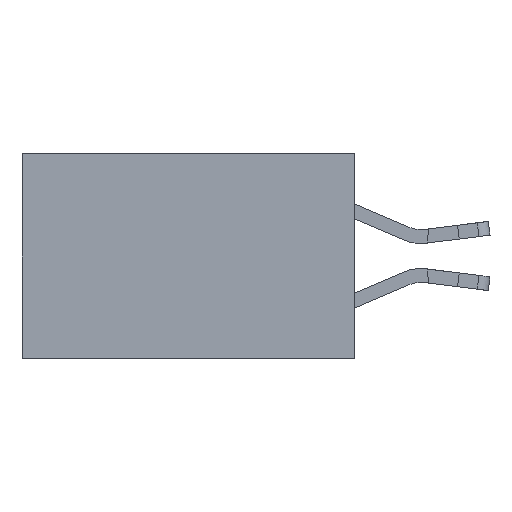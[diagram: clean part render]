
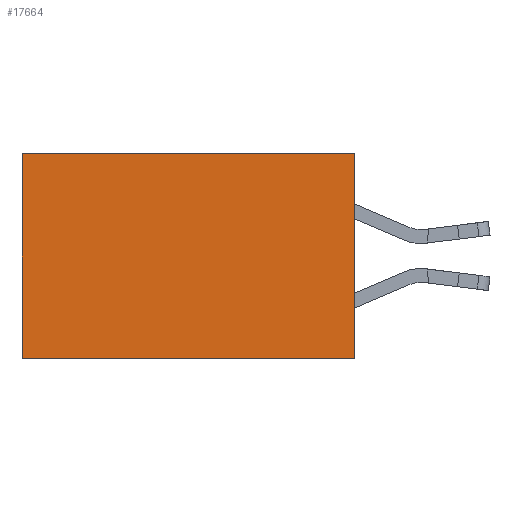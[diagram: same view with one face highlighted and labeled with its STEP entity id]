
A CAD part, left-side view. The second image highlights one B-rep face of the part: STEP entity #17664.
In plain terms, the highlighted planar face has unit normal (-1, 0, 0).
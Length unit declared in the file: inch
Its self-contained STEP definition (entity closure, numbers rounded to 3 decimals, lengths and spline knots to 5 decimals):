
#188 = VERTEX_POINT ( 'NONE', #12939 ) ;
#426 = VECTOR ( 'NONE', #7050, 39.37008 ) ;
#556 = CARTESIAN_POINT ( 'NONE',  ( 0.2615, 0., 0. ) ) ;
#1027 = EDGE_LOOP ( 'NONE', ( #6830, #12116, #4353, #14062 ) ) ;
#1072 = DIRECTION ( 'NONE',  ( 1., 0., 0. ) ) ;
#2561 = LINE ( 'NONE', #17749, #13215 ) ;
#3249 = DIRECTION ( 'NONE',  ( 0., 0., -1. ) ) ;
#3664 = EDGE_CURVE ( 'NONE', #188, #5093, #8620, .T. ) ;
#3828 = EDGE_CURVE ( 'NONE', #7345, #5093, #2561, .T. ) ;
#4353 = ORIENTED_EDGE ( 'NONE', *, *, #13419, .F. ) ;
#4537 = CARTESIAN_POINT ( 'NONE',  ( 0.2615, 0.6, -0.37 ) ) ;
#5093 = VERTEX_POINT ( 'NONE', #12777 ) ;
#6011 = AXIS2_PLACEMENT_3D ( 'NONE', #13455, #1072, #7748 ) ;
#6830 = ORIENTED_EDGE ( 'NONE', *, *, #3664, .T. ) ;
#7050 = DIRECTION ( 'NONE',  ( 0., 1., 0. ) ) ;
#7345 = VERTEX_POINT ( 'NONE', #13666 ) ;
#7748 = DIRECTION ( 'NONE',  ( 0., 0., -1. ) ) ;
#7937 = PLANE ( 'NONE',  #6011 ) ;
#8028 = FACE_OUTER_BOUND ( 'NONE', #1027, .T. ) ;
#8498 = CARTESIAN_POINT ( 'NONE',  ( 0.2615, 0., 0. ) ) ;
#8620 = LINE ( 'NONE', #4537, #17550 ) ;
#8813 = EDGE_CURVE ( 'NONE', #9346, #188, #10005, .T. ) ;
#9346 = VERTEX_POINT ( 'NONE', #556 ) ;
#10005 = LINE ( 'NONE', #8498, #426 ) ;
#10046 = DIRECTION ( 'NONE',  ( 0., 0., -1. ) ) ;
#10105 = LINE ( 'NONE', #15644, #13765 ) ;
#12116 = ORIENTED_EDGE ( 'NONE', *, *, #3828, .F. ) ;
#12777 = CARTESIAN_POINT ( 'NONE',  ( 0.2615, 0.6, -0.37 ) ) ;
#12939 = CARTESIAN_POINT ( 'NONE',  ( 0.2615, 0.6, 0. ) ) ;
#13215 = VECTOR ( 'NONE', #15053, 39.37008 ) ;
#13419 = EDGE_CURVE ( 'NONE', #9346, #7345, #10105, .T. ) ;
#13455 = CARTESIAN_POINT ( 'NONE',  ( 0.2615, 0., -0.37 ) ) ;
#13666 = CARTESIAN_POINT ( 'NONE',  ( 0.2615, 0., -0.37 ) ) ;
#13765 = VECTOR ( 'NONE', #3249, 39.37008 ) ;
#14062 = ORIENTED_EDGE ( 'NONE', *, *, #8813, .T. ) ;
#15053 = DIRECTION ( 'NONE',  ( 0., 1., 0. ) ) ;
#15644 = CARTESIAN_POINT ( 'NONE',  ( 0.2615, 0., -0.37 ) ) ;
#17550 = VECTOR ( 'NONE', #10046, 39.37008 ) ;
#17664 = ADVANCED_FACE ( 'NONE', ( #8028 ), #7937, .F. ) ;
#17749 = CARTESIAN_POINT ( 'NONE',  ( 0.2615, 0., -0.37 ) ) ;
